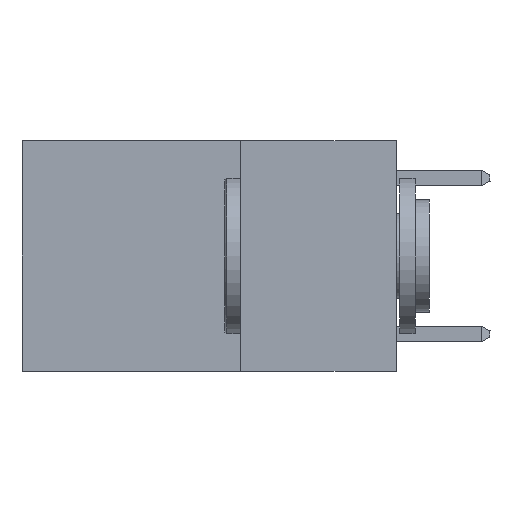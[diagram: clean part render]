
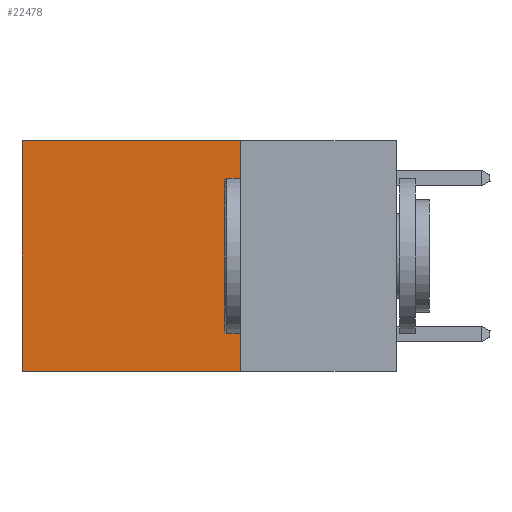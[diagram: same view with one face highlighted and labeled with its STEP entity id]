
A CAD part, left-side view. The second image highlights one B-rep face of the part: STEP entity #22478.
In plain terms, the highlighted planar face has unit normal (-1, 0, 0).
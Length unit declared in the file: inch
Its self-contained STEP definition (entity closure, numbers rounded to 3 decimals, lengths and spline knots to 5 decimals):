
#433 = CARTESIAN_POINT ( 'NONE',  ( 0.2625, 0.25, 0. ) ) ;
#1041 = CARTESIAN_POINT ( 'NONE',  ( 0.2625, 0.25, 0. ) ) ;
#1201 = DIRECTION ( 'NONE',  ( 0., 1., 0. ) ) ;
#1339 = VERTEX_POINT ( 'NONE', #22659 ) ;
#1826 = VECTOR ( 'NONE', #1201, 39.37008 ) ;
#4248 = AXIS2_PLACEMENT_3D ( 'NONE', #433, #12156, #14567 ) ;
#5933 = LINE ( 'NONE', #7927, #27166 ) ;
#6405 = VECTOR ( 'NONE', #10788, 39.37008 ) ;
#7326 = VECTOR ( 'NONE', #11221, 39.37008 ) ;
#7509 = ORIENTED_EDGE ( 'NONE', *, *, #27858, .F. ) ;
#7927 = CARTESIAN_POINT ( 'NONE',  ( 0.2625, 0.6, 0. ) ) ;
#8366 = DIRECTION ( 'NONE',  ( 0., 0., -1. ) ) ;
#8394 = EDGE_CURVE ( 'NONE', #1339, #14482, #5933, .T. ) ;
#10198 = CARTESIAN_POINT ( 'NONE',  ( 0.2625, 0.25, 0. ) ) ;
#10788 = DIRECTION ( 'NONE',  ( 0., 0., -1. ) ) ;
#11172 = VERTEX_POINT ( 'NONE', #27079 ) ;
#11221 = DIRECTION ( 'NONE',  ( 0., 1., 0. ) ) ;
#12156 = DIRECTION ( 'NONE',  ( 1., 0., 0. ) ) ;
#13073 = LINE ( 'NONE', #1041, #6405 ) ;
#14267 = EDGE_CURVE ( 'NONE', #11172, #14482, #29814, .T. ) ;
#14482 = VERTEX_POINT ( 'NONE', #20776 ) ;
#14567 = DIRECTION ( 'NONE',  ( 0., 0., -1. ) ) ;
#16033 = ORIENTED_EDGE ( 'NONE', *, *, #20774, .T. ) ;
#16039 = VERTEX_POINT ( 'NONE', #28893 ) ;
#20774 = EDGE_CURVE ( 'NONE', #16039, #1339, #21604, .T. ) ;
#20776 = CARTESIAN_POINT ( 'NONE',  ( 0.2625, 0.6, -0.37 ) ) ;
#21604 = LINE ( 'NONE', #10198, #1826 ) ;
#22478 = ADVANCED_FACE ( 'NONE', ( #26134 ), #27993, .F. ) ;
#22659 = CARTESIAN_POINT ( 'NONE',  ( 0.2625, 0.6, 0. ) ) ;
#24887 = CARTESIAN_POINT ( 'NONE',  ( 0.2625, 0.25, -0.37 ) ) ;
#25232 = EDGE_LOOP ( 'NONE', ( #29286, #28191, #7509, #16033 ) ) ;
#26134 = FACE_OUTER_BOUND ( 'NONE', #25232, .T. ) ;
#27079 = CARTESIAN_POINT ( 'NONE',  ( 0.2625, 0.25, -0.37 ) ) ;
#27166 = VECTOR ( 'NONE', #8366, 39.37008 ) ;
#27858 = EDGE_CURVE ( 'NONE', #16039, #11172, #13073, .T. ) ;
#27993 = PLANE ( 'NONE',  #4248 ) ;
#28191 = ORIENTED_EDGE ( 'NONE', *, *, #14267, .F. ) ;
#28893 = CARTESIAN_POINT ( 'NONE',  ( 0.2625, 0.25, 0. ) ) ;
#29286 = ORIENTED_EDGE ( 'NONE', *, *, #8394, .T. ) ;
#29814 = LINE ( 'NONE', #24887, #7326 ) ;
